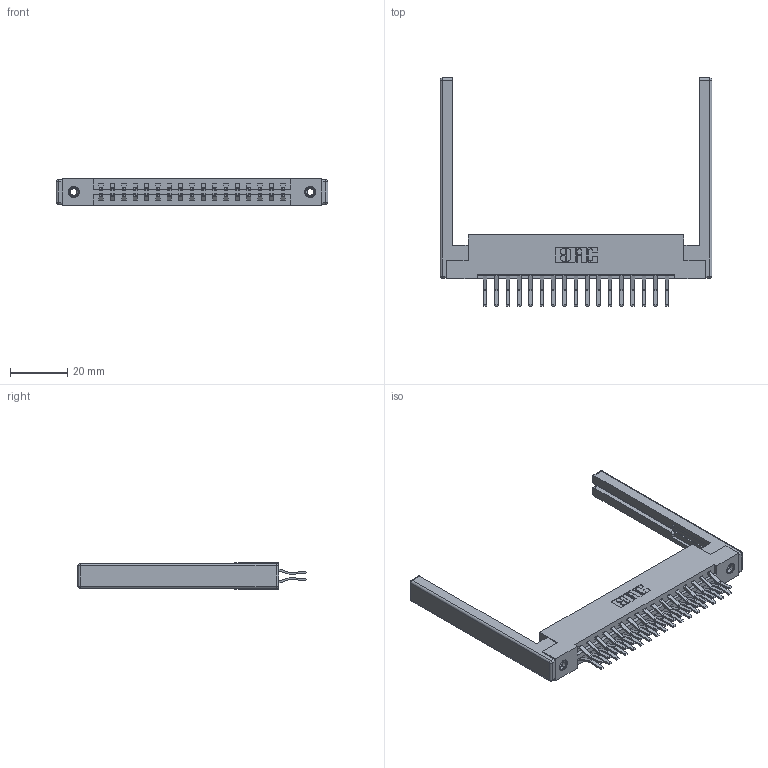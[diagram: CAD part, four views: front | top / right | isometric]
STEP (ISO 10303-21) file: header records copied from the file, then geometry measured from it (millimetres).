
FILE_DESCRIPTION (( 'STEP AP203' ), '1' );
FILE_NAME ('337-034-560-268.STEP', '2019-10-08T20:31:48', ( '' ), ( '' ), 'SwSTEP 2.0', 'SolidWorks 2016', '' );
FILE_SCHEMA (( 'CONFIG_CONTROL_DESIGN' ));
Length unit declared in the file: inch
Products named in the file (5): 307-220-068; 337-034-560-268; 345-292-001_560 Tail; 345-250-001_345-250-001-102; 337 Part_Flush Mounting Lugs - 0.156 Dia-TI
Assembly tree (39 placements, depth 2):
  337-034-560-268
    337 Part_Flush Mounting Lugs - 0.156 Dia-TI
    345-292-001_560 Tail  x34
    345-250-001_345-250-001-102  x2
    307-220-068  x2
Bounding box: 94.79 x 79.52 x 9.4 mm (x, y, z)
Volume: 14264.9 mm3; surface area: 15606 mm2
Topology: 39 solids, 39 shells, 2172 faces, 6379 edges, 4186 vertices
Faces by surface type: plane 1450, cylinder 698, cone 12, sphere 8, torus 4
Entity records: 19262 total; most frequent: CARTESIAN_POINT 3231, ORIENTED_EDGE 3156, DIRECTION 2868, EDGE_CURVE 1578, LINE 1396, VECTOR 1396, VERTEX_POINT 1042, AXIS2_PLACEMENT_3D 736
